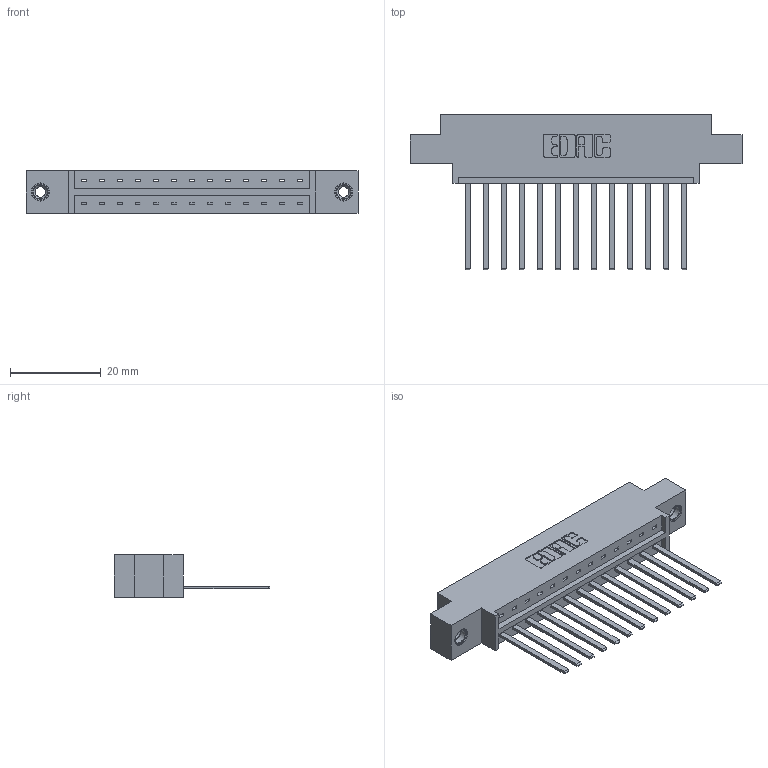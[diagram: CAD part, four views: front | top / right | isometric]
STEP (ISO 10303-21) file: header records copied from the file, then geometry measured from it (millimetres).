
FILE_DESCRIPTION (( 'STEP AP203' ), '1' );
FILE_NAME ('833-013-544-608.STEP', '2020-05-31T00:25:26', ( '' ), ( '' ), 'SwSTEP 2.0', 'SolidWorks 2020', '' );
FILE_SCHEMA (( 'CONFIG_CONTROL_DESIGN' ));
Length unit declared in the file: inch
Products named in the file (4): 833 Part_Offset - .156 Dia - TI; 345-292-001_345-293-144; 833-013-544-608; 345-250-001_345-250-003-102
Assembly tree (16 placements, depth 2):
  833-013-544-608
    833 Part_Offset - .156 Dia - TI
    345-292-001_345-293-144  x13
    345-250-001_345-250-003-102  x2
Bounding box: 73.05 x 34.3 x 9.4 mm (x, y, z)
Volume: 7017.8 mm3; surface area: 8116.7 mm2
Topology: 16 solids, 16 shells, 854 faces, 2513 edges, 1650 vertices
Faces by surface type: plane 600, cylinder 238, cone 12, torus 4
Entity records: 12832 total; most frequent: CARTESIAN_POINT 2200, ORIENTED_EDGE 2142, DIRECTION 1943, EDGE_CURVE 1071, VECTOR 927, LINE 927, VERTEX_POINT 708, AXIS2_PLACEMENT_3D 508
